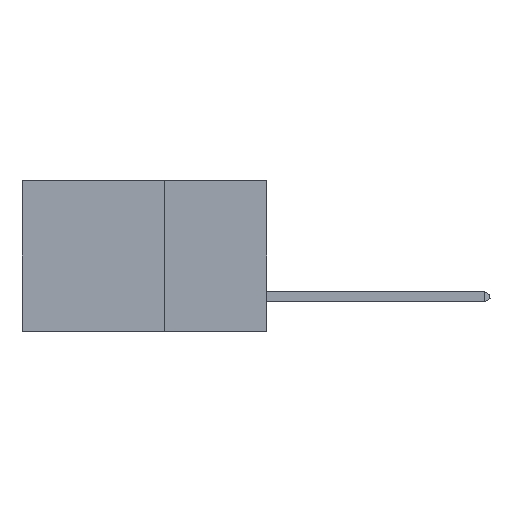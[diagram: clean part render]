
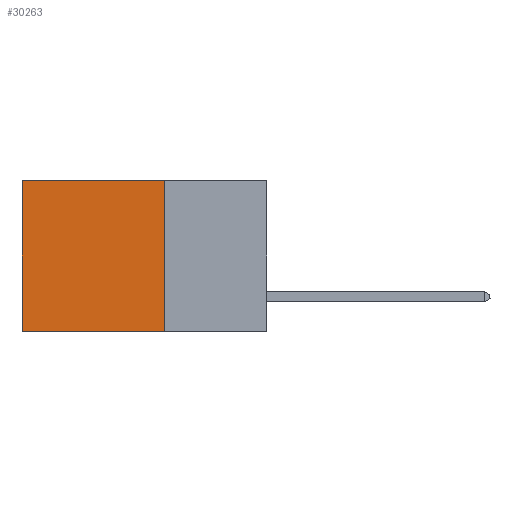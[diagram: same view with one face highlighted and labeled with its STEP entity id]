
A CAD part, left-side view. The second image highlights one B-rep face of the part: STEP entity #30263.
In plain terms, the highlighted planar face has unit normal (-1, 0, 0).
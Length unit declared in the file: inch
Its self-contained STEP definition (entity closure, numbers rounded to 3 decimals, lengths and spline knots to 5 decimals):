
#750 = ORIENTED_EDGE ( 'NONE', *, *, #25031, .F. ) ;
#1385 = CARTESIAN_POINT ( 'NONE',  ( 0.2875, 0.25, 0. ) ) ;
#3205 = DIRECTION ( 'NONE',  ( 1., 0., 0. ) ) ;
#4786 = LINE ( 'NONE', #15846, #23513 ) ;
#5082 = EDGE_CURVE ( 'NONE', #5396, #27132, #9697, .T. ) ;
#5287 = ORIENTED_EDGE ( 'NONE', *, *, #5082, .T. ) ;
#5396 = VERTEX_POINT ( 'NONE', #24275 ) ;
#5531 = VERTEX_POINT ( 'NONE', #1385 ) ;
#6100 = CARTESIAN_POINT ( 'NONE',  ( 0.2875, 0.6, 0. ) ) ;
#7888 = DIRECTION ( 'NONE',  ( 0., 0., -1. ) ) ;
#8312 = EDGE_LOOP ( 'NONE', ( #5287, #750, #23035, #22772 ) ) ;
#8602 = DIRECTION ( 'NONE',  ( 0., 1., 0. ) ) ;
#9144 = DIRECTION ( 'NONE',  ( 0., 0., -1. ) ) ;
#9697 = LINE ( 'NONE', #6100, #14277 ) ;
#13059 = DIRECTION ( 'NONE',  ( 0., 0., -1. ) ) ;
#13171 = CARTESIAN_POINT ( 'NONE',  ( 0.2875, 0.25, 0. ) ) ;
#13461 = VERTEX_POINT ( 'NONE', #21801 ) ;
#14277 = VECTOR ( 'NONE', #9144, 39.37008 ) ;
#14361 = VECTOR ( 'NONE', #7888, 39.37008 ) ;
#15021 = LINE ( 'NONE', #27497, #28350 ) ;
#15846 = CARTESIAN_POINT ( 'NONE',  ( 0.2875, 0.25, -0.37 ) ) ;
#16158 = CARTESIAN_POINT ( 'NONE',  ( 0.2875, 0.6, -0.37 ) ) ;
#17058 = EDGE_CURVE ( 'NONE', #5531, #5396, #15021, .T. ) ;
#19660 = LINE ( 'NONE', #24591, #14361 ) ;
#20806 = AXIS2_PLACEMENT_3D ( 'NONE', #13171, #3205, #13059 ) ;
#20907 = FACE_OUTER_BOUND ( 'NONE', #8312, .T. ) ;
#21801 = CARTESIAN_POINT ( 'NONE',  ( 0.2875, 0.25, -0.37 ) ) ;
#22772 = ORIENTED_EDGE ( 'NONE', *, *, #17058, .T. ) ;
#22922 = EDGE_CURVE ( 'NONE', #5531, #13461, #19660, .T. ) ;
#23035 = ORIENTED_EDGE ( 'NONE', *, *, #22922, .F. ) ;
#23513 = VECTOR ( 'NONE', #8602, 39.37008 ) ;
#24275 = CARTESIAN_POINT ( 'NONE',  ( 0.2875, 0.6, 0. ) ) ;
#24591 = CARTESIAN_POINT ( 'NONE',  ( 0.2875, 0.25, 0. ) ) ;
#25031 = EDGE_CURVE ( 'NONE', #13461, #27132, #4786, .T. ) ;
#25401 = PLANE ( 'NONE',  #20806 ) ;
#27132 = VERTEX_POINT ( 'NONE', #16158 ) ;
#27497 = CARTESIAN_POINT ( 'NONE',  ( 0.2875, 0.25, 0. ) ) ;
#28350 = VECTOR ( 'NONE', #29736, 39.37008 ) ;
#29736 = DIRECTION ( 'NONE',  ( 0., 1., 0. ) ) ;
#30263 = ADVANCED_FACE ( 'NONE', ( #20907 ), #25401, .F. ) ;
